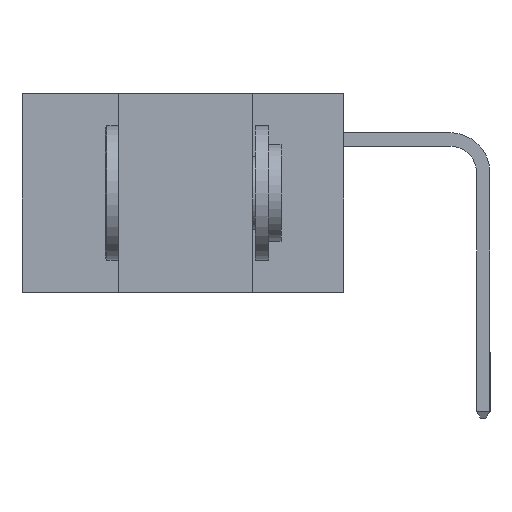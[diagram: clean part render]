
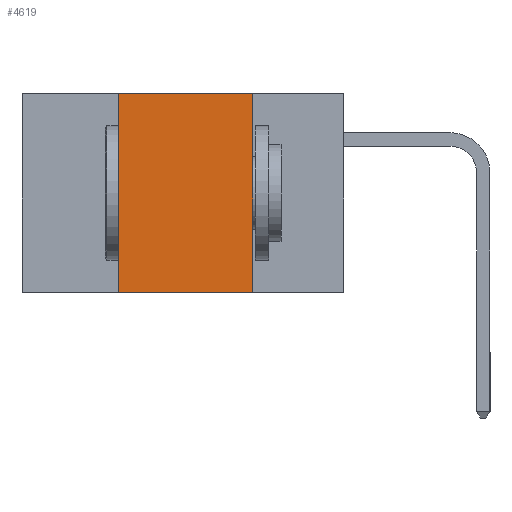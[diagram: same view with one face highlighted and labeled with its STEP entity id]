
A CAD part, left-side view. The second image highlights one B-rep face of the part: STEP entity #4619.
In plain terms, the highlighted planar face has unit normal (-1, 0, 0).
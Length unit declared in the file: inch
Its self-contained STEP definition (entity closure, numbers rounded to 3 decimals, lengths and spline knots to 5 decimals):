
#218 = ORIENTED_EDGE ( 'NONE', *, *, #5759, .T. ) ;
#784 = ORIENTED_EDGE ( 'NONE', *, *, #8318, .F. ) ;
#814 = CARTESIAN_POINT ( 'NONE',  ( 0., 0.42, 0. ) ) ;
#834 = EDGE_CURVE ( 'NONE', #2514, #4083, #1517, .T. ) ;
#1103 = CARTESIAN_POINT ( 'NONE',  ( 0., 0.6, 0. ) ) ;
#1167 = DIRECTION ( 'NONE',  ( 0., -1., 0. ) ) ;
#1499 = CARTESIAN_POINT ( 'NONE',  ( 0., 0.42, -0.37 ) ) ;
#1517 = LINE ( 'NONE', #5409, #9854 ) ;
#1638 = DIRECTION ( 'NONE',  ( 0., 0., 1. ) ) ;
#1653 = VECTOR ( 'NONE', #6605, 39.37008 ) ;
#2000 = FACE_OUTER_BOUND ( 'NONE', #6527, .T. ) ;
#2188 = DIRECTION ( 'NONE',  ( 1., 0., 0. ) ) ;
#2514 = VERTEX_POINT ( 'NONE', #1499 ) ;
#2638 = CARTESIAN_POINT ( 'NONE',  ( 0., 0.17, 0. ) ) ;
#2841 = EDGE_CURVE ( 'NONE', #4083, #9687, #9840, .T. ) ;
#4083 = VERTEX_POINT ( 'NONE', #814 ) ;
#4226 = VECTOR ( 'NONE', #1167, 39.37008 ) ;
#4619 = ADVANCED_FACE ( 'NONE', ( #2000 ), #5048, .F. ) ;
#5048 = PLANE ( 'NONE',  #8779 ) ;
#5274 = CARTESIAN_POINT ( 'NONE',  ( 0., 0.17, -0.37 ) ) ;
#5396 = DIRECTION ( 'NONE',  ( 0., 0., -1. ) ) ;
#5409 = CARTESIAN_POINT ( 'NONE',  ( 0., 0.42, -0.37 ) ) ;
#5759 = EDGE_CURVE ( 'NONE', #2514, #6647, #11626, .T. ) ;
#5772 = ORIENTED_EDGE ( 'NONE', *, *, #2841, .F. ) ;
#6159 = LINE ( 'NONE', #5274, #9234 ) ;
#6527 = EDGE_LOOP ( 'NONE', ( #784, #5772, #7290, #218 ) ) ;
#6605 = DIRECTION ( 'NONE',  ( 0., -1., 0. ) ) ;
#6647 = VERTEX_POINT ( 'NONE', #9374 ) ;
#7290 = ORIENTED_EDGE ( 'NONE', *, *, #834, .F. ) ;
#8318 = EDGE_CURVE ( 'NONE', #9687, #6647, #6159, .T. ) ;
#8634 = CARTESIAN_POINT ( 'NONE',  ( 0., 0.6, -0.37 ) ) ;
#8779 = AXIS2_PLACEMENT_3D ( 'NONE', #9910, #2188, #10735 ) ;
#9234 = VECTOR ( 'NONE', #5396, 39.37008 ) ;
#9374 = CARTESIAN_POINT ( 'NONE',  ( 0., 0.17, -0.37 ) ) ;
#9687 = VERTEX_POINT ( 'NONE', #2638 ) ;
#9840 = LINE ( 'NONE', #1103, #4226 ) ;
#9854 = VECTOR ( 'NONE', #1638, 39.37008 ) ;
#9910 = CARTESIAN_POINT ( 'NONE',  ( 0., 0.6, 0. ) ) ;
#10735 = DIRECTION ( 'NONE',  ( 0., 0., -1. ) ) ;
#11626 = LINE ( 'NONE', #8634, #1653 ) ;
